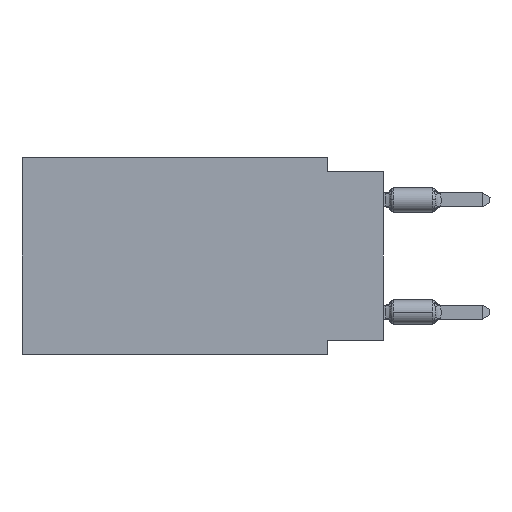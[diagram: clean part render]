
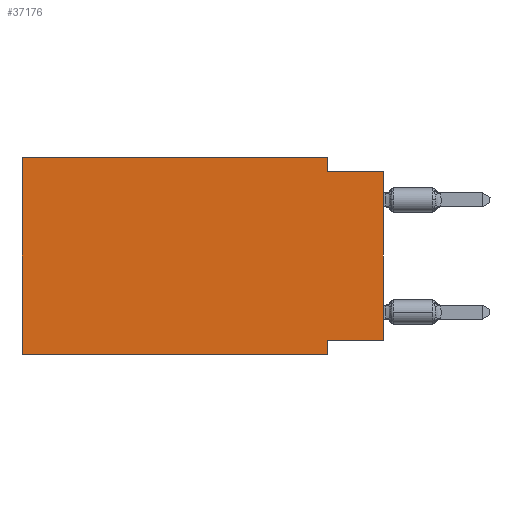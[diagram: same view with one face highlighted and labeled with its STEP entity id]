
A CAD part, left-side view. The second image highlights one B-rep face of the part: STEP entity #37176.
In plain terms, the highlighted planar face has unit normal (-1, 0, 0).
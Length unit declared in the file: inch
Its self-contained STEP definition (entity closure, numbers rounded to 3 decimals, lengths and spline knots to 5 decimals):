
#391 = LINE ( 'NONE', #32491, #20552 ) ;
#505 = CARTESIAN_POINT ( 'NONE',  ( 0., 0., -0.025 ) ) ;
#1865 = LINE ( 'NONE', #24533, #2972 ) ;
#2972 = VECTOR ( 'NONE', #21889, 39.37008 ) ;
#3659 = VERTEX_POINT ( 'NONE', #17154 ) ;
#4198 = EDGE_CURVE ( 'NONE', #19841, #16797, #21453, .T. ) ;
#5813 = DIRECTION ( 'NONE',  ( 0., -1., 0. ) ) ;
#6582 = VECTOR ( 'NONE', #10405, 39.37008 ) ;
#6734 = VECTOR ( 'NONE', #19479, 39.37008 ) ;
#6854 = ORIENTED_EDGE ( 'NONE', *, *, #31039, .T. ) ;
#7365 = AXIS2_PLACEMENT_3D ( 'NONE', #23517, #29382, #12374 ) ;
#7464 = ORIENTED_EDGE ( 'NONE', *, *, #4198, .F. ) ;
#8167 = VERTEX_POINT ( 'NONE', #28372 ) ;
#8832 = CARTESIAN_POINT ( 'NONE',  ( 0., 0.645, 0. ) ) ;
#9750 = LINE ( 'NONE', #505, #24136 ) ;
#9875 = LINE ( 'NONE', #21410, #6734 ) ;
#10405 = DIRECTION ( 'NONE',  ( 0., 0., -1. ) ) ;
#10548 = ORIENTED_EDGE ( 'NONE', *, *, #21296, .T. ) ;
#10862 = CARTESIAN_POINT ( 'NONE',  ( 0., 0., -0.325 ) ) ;
#11438 = CARTESIAN_POINT ( 'NONE',  ( 0., 0., -0.025 ) ) ;
#11827 = LINE ( 'NONE', #34683, #35948 ) ;
#12001 = EDGE_LOOP ( 'NONE', ( #6854, #35520, #12686, #15939, #31203, #10548, #24197, #7464 ) ) ;
#12374 = DIRECTION ( 'NONE',  ( 0., 0., -1. ) ) ;
#12686 = ORIENTED_EDGE ( 'NONE', *, *, #14879, .F. ) ;
#13308 = VERTEX_POINT ( 'NONE', #11438 ) ;
#13678 = CARTESIAN_POINT ( 'NONE',  ( 0., 0.645, -0.35 ) ) ;
#14879 = EDGE_CURVE ( 'NONE', #26016, #19272, #30252, .T. ) ;
#15436 = DIRECTION ( 'NONE',  ( 0., -1., 0. ) ) ;
#15939 = ORIENTED_EDGE ( 'NONE', *, *, #32792, .F. ) ;
#16797 = VERTEX_POINT ( 'NONE', #28619 ) ;
#17154 = CARTESIAN_POINT ( 'NONE',  ( 0., 0.645, 0. ) ) ;
#17809 = CARTESIAN_POINT ( 'NONE',  ( 0., 0.1, 0. ) ) ;
#18667 = EDGE_CURVE ( 'NONE', #16797, #8167, #391, .T. ) ;
#19272 = VERTEX_POINT ( 'NONE', #26989 ) ;
#19479 = DIRECTION ( 'NONE',  ( 0., 0., 1. ) ) ;
#19841 = VERTEX_POINT ( 'NONE', #10862 ) ;
#20552 = VECTOR ( 'NONE', #32671, 39.37008 ) ;
#21296 = EDGE_CURVE ( 'NONE', #22942, #8167, #1865, .T. ) ;
#21410 = CARTESIAN_POINT ( 'NONE',  ( 0., 0.645, 0. ) ) ;
#21453 = LINE ( 'NONE', #32944, #29115 ) ;
#21889 = DIRECTION ( 'NONE',  ( 0., -1., 0. ) ) ;
#22942 = VERTEX_POINT ( 'NONE', #13678 ) ;
#23517 = CARTESIAN_POINT ( 'NONE',  ( 0., 0.645, 0. ) ) ;
#24076 = PLANE ( 'NONE',  #7365 ) ;
#24136 = VECTOR ( 'NONE', #15436, 39.37008 ) ;
#24197 = ORIENTED_EDGE ( 'NONE', *, *, #18667, .F. ) ;
#24531 = EDGE_CURVE ( 'NONE', #19272, #13308, #9750, .T. ) ;
#24533 = CARTESIAN_POINT ( 'NONE',  ( 0., 0.645, -0.35 ) ) ;
#26016 = VERTEX_POINT ( 'NONE', #17809 ) ;
#26952 = DIRECTION ( 'NONE',  ( 0., 1., 0. ) ) ;
#26989 = CARTESIAN_POINT ( 'NONE',  ( 0., 0.1, -0.025 ) ) ;
#27609 = CARTESIAN_POINT ( 'NONE',  ( 0., 0.1, 0. ) ) ;
#28372 = CARTESIAN_POINT ( 'NONE',  ( 0., 0.1, -0.35 ) ) ;
#28619 = CARTESIAN_POINT ( 'NONE',  ( 0., 0.1, -0.325 ) ) ;
#29115 = VECTOR ( 'NONE', #26952, 39.37008 ) ;
#29382 = DIRECTION ( 'NONE',  ( 1., 0., 0. ) ) ;
#30252 = LINE ( 'NONE', #27609, #6582 ) ;
#31039 = EDGE_CURVE ( 'NONE', #19841, #13308, #11827, .T. ) ;
#31203 = ORIENTED_EDGE ( 'NONE', *, *, #36188, .F. ) ;
#32433 = LINE ( 'NONE', #8832, #35445 ) ;
#32491 = CARTESIAN_POINT ( 'NONE',  ( 0., 0.1, -0.35 ) ) ;
#32671 = DIRECTION ( 'NONE',  ( 0., 0., -1. ) ) ;
#32792 = EDGE_CURVE ( 'NONE', #3659, #26016, #32433, .T. ) ;
#32933 = FACE_OUTER_BOUND ( 'NONE', #12001, .T. ) ;
#32944 = CARTESIAN_POINT ( 'NONE',  ( 0., 0., -0.325 ) ) ;
#34683 = CARTESIAN_POINT ( 'NONE',  ( 0., 0., 0. ) ) ;
#34866 = DIRECTION ( 'NONE',  ( 0., 0., 1. ) ) ;
#35445 = VECTOR ( 'NONE', #5813, 39.37008 ) ;
#35520 = ORIENTED_EDGE ( 'NONE', *, *, #24531, .F. ) ;
#35948 = VECTOR ( 'NONE', #34866, 39.37008 ) ;
#36188 = EDGE_CURVE ( 'NONE', #22942, #3659, #9875, .T. ) ;
#37176 = ADVANCED_FACE ( 'NONE', ( #32933 ), #24076, .F. ) ;
